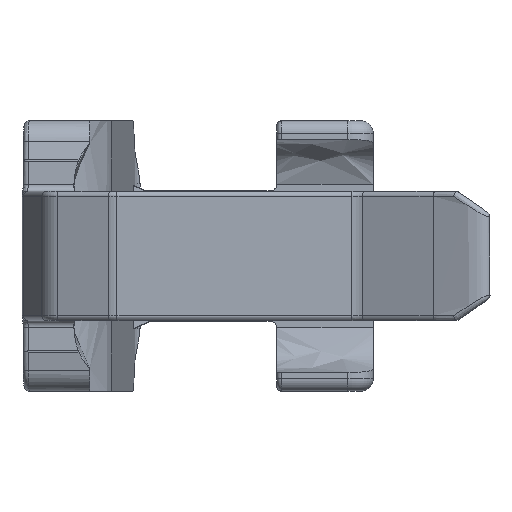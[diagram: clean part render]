
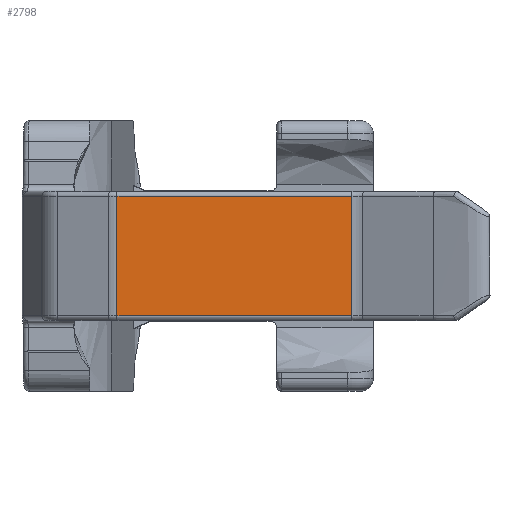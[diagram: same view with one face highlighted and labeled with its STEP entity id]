
A CAD part, left-side view. The second image highlights one B-rep face of the part: STEP entity #2798.
In plain terms, the highlighted planar face has unit normal (-1, 0, 0).
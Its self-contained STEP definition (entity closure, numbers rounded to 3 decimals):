
#205 = DIRECTION ( 'NONE',  ( 0., -1., 0. ) ) ;
#338 = CARTESIAN_POINT ( 'NONE',  ( -36.507, 2.923, 0. ) ) ;
#410 = ORIENTED_EDGE ( 'NONE', *, *, #1217, .T. ) ;
#565 = LINE ( 'NONE', #4515, #4266 ) ;
#843 = VECTOR ( 'NONE', #1800, 1000. ) ;
#851 = VECTOR ( 'NONE', #4967, 1000. ) ;
#1217 = EDGE_CURVE ( 'NONE', #2390, #2497, #2072, .T. ) ;
#1568 = DIRECTION ( 'NONE',  ( 0., -1., 0. ) ) ;
#1593 = VECTOR ( 'NONE', #2137, 1000. ) ;
#1688 = EDGE_CURVE ( 'NONE', #3347, #4730, #565, .T. ) ;
#1709 = CARTESIAN_POINT ( 'NONE',  ( -36.507, 21.423, 15.35 ) ) ;
#1800 = DIRECTION ( 'NONE',  ( 0., 0., 1. ) ) ;
#1810 = EDGE_LOOP ( 'NONE', ( #6137, #4390, #2852, #410 ) ) ;
#2072 = LINE ( 'NONE', #2668, #1593 ) ;
#2137 = DIRECTION ( 'NONE',  ( 0., 1., 0. ) ) ;
#2390 = VERTEX_POINT ( 'NONE', #5560 ) ;
#2497 = VERTEX_POINT ( 'NONE', #1709 ) ;
#2552 = CARTESIAN_POINT ( 'NONE',  ( -36.507, 2.923, 0. ) ) ;
#2561 = EDGE_CURVE ( 'NONE', #4730, #2390, #4654, .T. ) ;
#2668 = CARTESIAN_POINT ( 'NONE',  ( -36.507, 21.423, 15.35 ) ) ;
#2798 = ADVANCED_FACE ( 'NONE', ( #5445 ), #3461, .F. ) ;
#2852 = ORIENTED_EDGE ( 'NONE', *, *, #2561, .T. ) ;
#3055 = CARTESIAN_POINT ( 'NONE',  ( -36.507, 21.423, 0. ) ) ;
#3347 = VERTEX_POINT ( 'NONE', #5064 ) ;
#3461 = PLANE ( 'NONE',  #5974 ) ;
#3963 = DIRECTION ( 'NONE',  ( 1., 0., 0. ) ) ;
#4194 = EDGE_CURVE ( 'NONE', #3347, #2497, #5447, .T. ) ;
#4266 = VECTOR ( 'NONE', #205, 1000. ) ;
#4390 = ORIENTED_EDGE ( 'NONE', *, *, #1688, .T. ) ;
#4515 = CARTESIAN_POINT ( 'NONE',  ( -36.507, 2.923, 5.95 ) ) ;
#4654 = LINE ( 'NONE', #338, #843 ) ;
#4660 = CARTESIAN_POINT ( 'NONE',  ( -36.507, 2.923, 5.95 ) ) ;
#4730 = VERTEX_POINT ( 'NONE', #4660 ) ;
#4967 = DIRECTION ( 'NONE',  ( 0., 0., 1. ) ) ;
#5064 = CARTESIAN_POINT ( 'NONE',  ( -36.507, 21.423, 5.95 ) ) ;
#5445 = FACE_OUTER_BOUND ( 'NONE', #1810, .T. ) ;
#5447 = LINE ( 'NONE', #3055, #851 ) ;
#5560 = CARTESIAN_POINT ( 'NONE',  ( -36.507, 2.923, 15.35 ) ) ;
#5974 = AXIS2_PLACEMENT_3D ( 'NONE', #2552, #3963, #1568 ) ;
#6137 = ORIENTED_EDGE ( 'NONE', *, *, #4194, .F. ) ;
